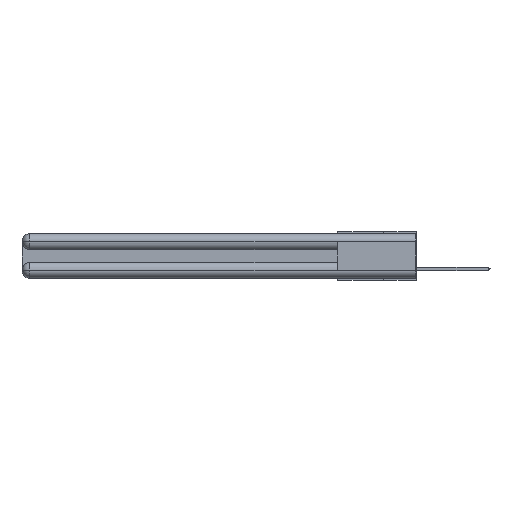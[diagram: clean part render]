
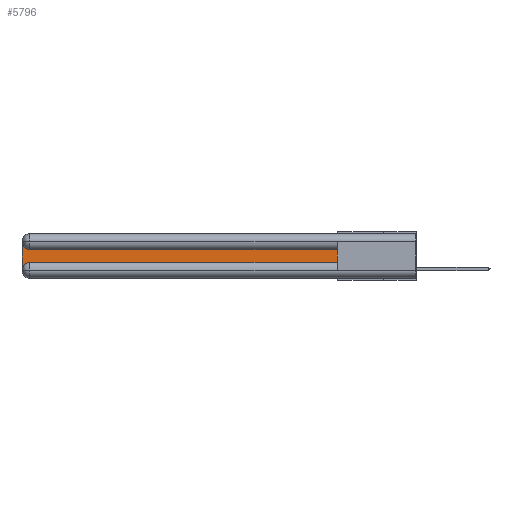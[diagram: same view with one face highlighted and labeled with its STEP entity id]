
A CAD part, left-side view. The second image highlights one B-rep face of the part: STEP entity #5796.
In plain terms, the highlighted planar face has unit normal (-1, 0, 0).
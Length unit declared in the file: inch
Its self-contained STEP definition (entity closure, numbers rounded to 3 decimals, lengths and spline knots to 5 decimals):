
#1119 = DIRECTION ( 'NONE',  ( 0., 0., -1. ) ) ;
#1692 = CIRCLE ( 'NONE', #15450, 0.06 ) ;
#1928 = PLANE ( 'NONE',  #6393 ) ;
#2696 = ORIENTED_EDGE ( 'NONE', *, *, #21880, .T. ) ;
#2783 = LINE ( 'NONE', #17083, #4836 ) ;
#3491 = DIRECTION ( 'NONE',  ( 0., 0., -1. ) ) ;
#3587 = DIRECTION ( 'NONE',  ( 0., -1., 0. ) ) ;
#4162 = VERTEX_POINT ( 'NONE', #13318 ) ;
#4189 = EDGE_CURVE ( 'NONE', #19279, #22972, #15307, .T. ) ;
#4836 = VECTOR ( 'NONE', #3587, 39.37008 ) ;
#5796 = ADVANCED_FACE ( 'NONE', ( #19623 ), #1928, .F. ) ;
#6393 = AXIS2_PLACEMENT_3D ( 'NONE', #19813, #27691, #7249 ) ;
#6747 = VECTOR ( 'NONE', #7067, 39.37008 ) ;
#6857 = ORIENTED_EDGE ( 'NONE', *, *, #27882, .T. ) ;
#7067 = DIRECTION ( 'NONE',  ( 0., 1., 0. ) ) ;
#7249 = DIRECTION ( 'NONE',  ( 0., 0., -1. ) ) ;
#8063 = CARTESIAN_POINT ( 'NONE',  ( 0.075, 0.6, -0.2175 ) ) ;
#8346 = EDGE_CURVE ( 'NONE', #30417, #13380, #28424, .T. ) ;
#9715 = ORIENTED_EDGE ( 'NONE', *, *, #26060, .T. ) ;
#10238 = CARTESIAN_POINT ( 'NONE',  ( 0.075, 0.6, -0.1225 ) ) ;
#11086 = CARTESIAN_POINT ( 'NONE',  ( 0.075, 2.94, -0.0625 ) ) ;
#13043 = EDGE_CURVE ( 'NONE', #13380, #19279, #2783, .T. ) ;
#13195 = DIRECTION ( 'NONE',  ( 0., 0., 1. ) ) ;
#13318 = CARTESIAN_POINT ( 'NONE',  ( 0.075, 3., -0.0625 ) ) ;
#13380 = VERTEX_POINT ( 'NONE', #18868 ) ;
#13615 = VERTEX_POINT ( 'NONE', #29175 ) ;
#15307 = LINE ( 'NONE', #8063, #32459 ) ;
#15450 = AXIS2_PLACEMENT_3D ( 'NONE', #11086, #18661, #31441 ) ;
#17083 = CARTESIAN_POINT ( 'NONE',  ( 0.075, 0.6, -0.2175 ) ) ;
#18661 = DIRECTION ( 'NONE',  ( 1., 0., 0. ) ) ;
#18868 = CARTESIAN_POINT ( 'NONE',  ( 0.075, 2.94, -0.2175 ) ) ;
#19279 = VERTEX_POINT ( 'NONE', #21472 ) ;
#19623 = FACE_OUTER_BOUND ( 'NONE', #26408, .T. ) ;
#19813 = CARTESIAN_POINT ( 'NONE',  ( 0.075, 3., -0.1225 ) ) ;
#20838 = VECTOR ( 'NONE', #1119, 39.37008 ) ;
#21307 = ORIENTED_EDGE ( 'NONE', *, *, #4189, .T. ) ;
#21472 = CARTESIAN_POINT ( 'NONE',  ( 0.075, 0.6, -0.2175 ) ) ;
#21880 = EDGE_CURVE ( 'NONE', #13615, #4162, #1692, .T. ) ;
#22972 = VERTEX_POINT ( 'NONE', #10238 ) ;
#23243 = CARTESIAN_POINT ( 'NONE',  ( 0.075, 3., -0.2775 ) ) ;
#23608 = ORIENTED_EDGE ( 'NONE', *, *, #13043, .T. ) ;
#23925 = AXIS2_PLACEMENT_3D ( 'NONE', #26613, #29718, #3491 ) ;
#23969 = ORIENTED_EDGE ( 'NONE', *, *, #8346, .T. ) ;
#24102 = LINE ( 'NONE', #24444, #20838 ) ;
#24444 = CARTESIAN_POINT ( 'NONE',  ( 0.075, 3., -0.2175 ) ) ;
#25965 = LINE ( 'NONE', #28415, #6747 ) ;
#26060 = EDGE_CURVE ( 'NONE', #4162, #30417, #24102, .T. ) ;
#26408 = EDGE_LOOP ( 'NONE', ( #6857, #2696, #9715, #23969, #23608, #21307 ) ) ;
#26613 = CARTESIAN_POINT ( 'NONE',  ( 0.075, 2.94, -0.2775 ) ) ;
#27691 = DIRECTION ( 'NONE',  ( 1., 0., 0. ) ) ;
#27882 = EDGE_CURVE ( 'NONE', #22972, #13615, #25965, .T. ) ;
#28415 = CARTESIAN_POINT ( 'NONE',  ( 0.075, 0.6, -0.1225 ) ) ;
#28424 = CIRCLE ( 'NONE', #23925, 0.06 ) ;
#29175 = CARTESIAN_POINT ( 'NONE',  ( 0.075, 2.94, -0.1225 ) ) ;
#29718 = DIRECTION ( 'NONE',  ( 1., 0., 0. ) ) ;
#30417 = VERTEX_POINT ( 'NONE', #23243 ) ;
#31441 = DIRECTION ( 'NONE',  ( 0., 0., -1. ) ) ;
#32459 = VECTOR ( 'NONE', #13195, 39.37008 ) ;
